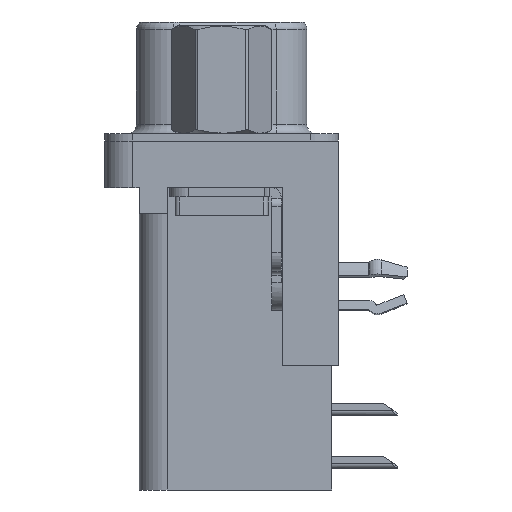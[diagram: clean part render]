
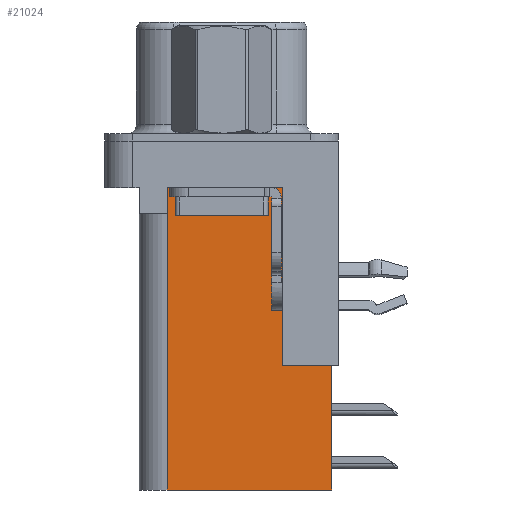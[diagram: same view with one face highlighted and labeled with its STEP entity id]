
A CAD part, left-side view. The second image highlights one B-rep face of the part: STEP entity #21024.
In plain terms, the highlighted planar face has unit normal (-1, 0, 0).
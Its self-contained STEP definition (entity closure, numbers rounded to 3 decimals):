
#983 = DIRECTION ( 'NONE',  ( 0., 1., 0. ) ) ;
#1155 = DIRECTION ( 'NONE',  ( 0., 1., 0. ) ) ;
#1221 = EDGE_LOOP ( 'NONE', ( #11581, #17508, #3054, #11387, #14536, #14362, #13548, #22354 ) ) ;
#1650 = EDGE_CURVE ( 'NONE', #22378, #10442, #12012, .T. ) ;
#1977 = CARTESIAN_POINT ( 'NONE',  ( 3.79, -5.925, -12.05 ) ) ;
#3054 = ORIENTED_EDGE ( 'NONE', *, *, #6428, .T. ) ;
#3117 = VECTOR ( 'NONE', #7279, 1000. ) ;
#3437 = VECTOR ( 'NONE', #1155, 1000. ) ;
#3450 = CARTESIAN_POINT ( 'NONE',  ( 3.79, 2.895, -3.9 ) ) ;
#4121 = CARTESIAN_POINT ( 'NONE',  ( 3.79, -3.295, -18.76 ) ) ;
#5132 = VERTEX_POINT ( 'NONE', #19755 ) ;
#5431 = LINE ( 'NONE', #3450, #9058 ) ;
#5584 = CARTESIAN_POINT ( 'NONE',  ( 3.79, -5.925, -18.76 ) ) ;
#5782 = VERTEX_POINT ( 'NONE', #15564 ) ;
#6428 = EDGE_CURVE ( 'NONE', #11244, #20942, #7927, .T. ) ;
#7038 = CARTESIAN_POINT ( 'NONE',  ( 3.79, -3.295, -18.76 ) ) ;
#7279 = DIRECTION ( 'NONE',  ( 0., 1., 0. ) ) ;
#7671 = LINE ( 'NONE', #20783, #20598 ) ;
#7688 = DIRECTION ( 'NONE',  ( 0., 0., -1. ) ) ;
#7927 = LINE ( 'NONE', #10805, #3117 ) ;
#8220 = LINE ( 'NONE', #13644, #3437 ) ;
#8838 = DIRECTION ( 'NONE',  ( 0., 1., 0. ) ) ;
#8967 = EDGE_CURVE ( 'NONE', #10496, #5782, #8220, .T. ) ;
#9005 = EDGE_CURVE ( 'NONE', #10442, #20942, #7671, .T. ) ;
#9058 = VECTOR ( 'NONE', #10618, 1000. ) ;
#9344 = FACE_OUTER_BOUND ( 'NONE', #1221, .T. ) ;
#9669 = CARTESIAN_POINT ( 'NONE',  ( 3.79, 2.895, -3.9 ) ) ;
#9709 = CARTESIAN_POINT ( 'NONE',  ( 3.79, -3.295, -2.5 ) ) ;
#10442 = VERTEX_POINT ( 'NONE', #16643 ) ;
#10446 = VECTOR ( 'NONE', #21583, 1000. ) ;
#10496 = VERTEX_POINT ( 'NONE', #9709 ) ;
#10618 = DIRECTION ( 'NONE',  ( 0., 0., -1. ) ) ;
#10805 = CARTESIAN_POINT ( 'NONE',  ( 3.79, 0., -3.9 ) ) ;
#11062 = AXIS2_PLACEMENT_3D ( 'NONE', #7038, #19389, #8838 ) ;
#11115 = CARTESIAN_POINT ( 'NONE',  ( 3.79, -6.295, -12.05 ) ) ;
#11244 = VERTEX_POINT ( 'NONE', #9669 ) ;
#11387 = ORIENTED_EDGE ( 'NONE', *, *, #9005, .F. ) ;
#11581 = ORIENTED_EDGE ( 'NONE', *, *, #8967, .T. ) ;
#12012 = LINE ( 'NONE', #15554, #16703 ) ;
#13456 = VECTOR ( 'NONE', #16531, 1000. ) ;
#13548 = ORIENTED_EDGE ( 'NONE', *, *, #22947, .T. ) ;
#13644 = CARTESIAN_POINT ( 'NONE',  ( 3.79, -3.295, -2.5 ) ) ;
#14362 = ORIENTED_EDGE ( 'NONE', *, *, #14663, .F. ) ;
#14536 = ORIENTED_EDGE ( 'NONE', *, *, #1650, .F. ) ;
#14663 = EDGE_CURVE ( 'NONE', #21220, #22378, #16575, .T. ) ;
#15093 = LINE ( 'NONE', #11115, #10446 ) ;
#15205 = CARTESIAN_POINT ( 'NONE',  ( 3.79, 2.925, -3.9 ) ) ;
#15554 = CARTESIAN_POINT ( 'NONE',  ( 3.79, -3.295, -18.76 ) ) ;
#15564 = CARTESIAN_POINT ( 'NONE',  ( 3.79, 2.895, -2.5 ) ) ;
#16531 = DIRECTION ( 'NONE',  ( 0., 0., 1. ) ) ;
#16575 = LINE ( 'NONE', #21677, #17126 ) ;
#16609 = EDGE_CURVE ( 'NONE', #5132, #10496, #18710, .T. ) ;
#16643 = CARTESIAN_POINT ( 'NONE',  ( 3.79, 2.925, -18.76 ) ) ;
#16703 = VECTOR ( 'NONE', #983, 1000. ) ;
#17043 = EDGE_CURVE ( 'NONE', #5782, #11244, #5431, .T. ) ;
#17126 = VECTOR ( 'NONE', #7688, 1000. ) ;
#17157 = PLANE ( 'NONE',  #11062 ) ;
#17508 = ORIENTED_EDGE ( 'NONE', *, *, #17043, .T. ) ;
#18710 = LINE ( 'NONE', #4121, #13456 ) ;
#19389 = DIRECTION ( 'NONE',  ( 1., 0., 0. ) ) ;
#19755 = CARTESIAN_POINT ( 'NONE',  ( 3.79, -3.295, -12.05 ) ) ;
#20598 = VECTOR ( 'NONE', #20637, 1000. ) ;
#20637 = DIRECTION ( 'NONE',  ( 0., 0., 1. ) ) ;
#20783 = CARTESIAN_POINT ( 'NONE',  ( 3.79, 2.925, -18.76 ) ) ;
#20942 = VERTEX_POINT ( 'NONE', #15205 ) ;
#21024 = ADVANCED_FACE ( 'NONE', ( #9344 ), #17157, .F. ) ;
#21220 = VERTEX_POINT ( 'NONE', #1977 ) ;
#21583 = DIRECTION ( 'NONE',  ( 0., 1., 0. ) ) ;
#21677 = CARTESIAN_POINT ( 'NONE',  ( 3.79, -5.925, -2. ) ) ;
#22354 = ORIENTED_EDGE ( 'NONE', *, *, #16609, .T. ) ;
#22378 = VERTEX_POINT ( 'NONE', #5584 ) ;
#22947 = EDGE_CURVE ( 'NONE', #21220, #5132, #15093, .T. ) ;
